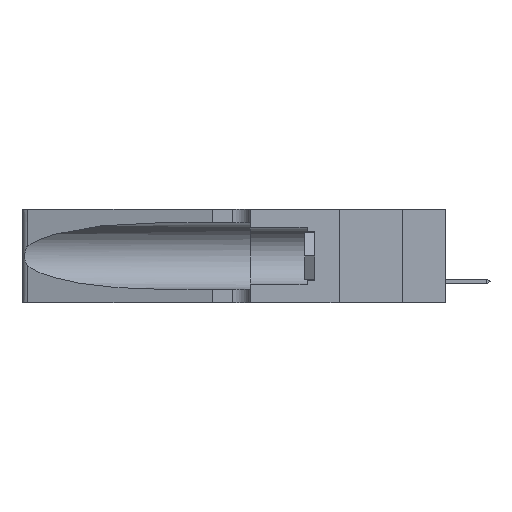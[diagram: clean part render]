
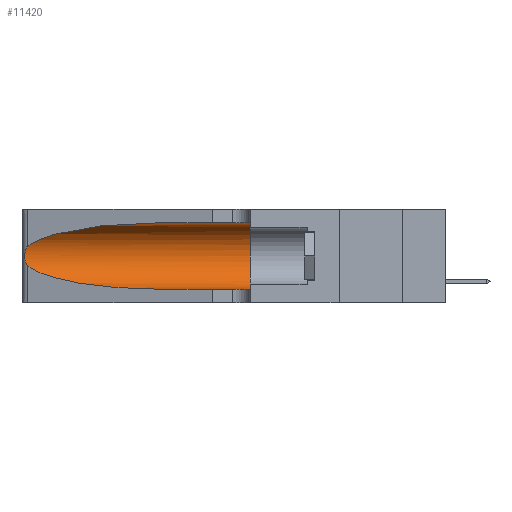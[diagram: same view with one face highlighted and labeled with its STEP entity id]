
A CAD part, left-side view. The second image highlights one B-rep face of the part: STEP entity #11420.
In plain terms, the highlighted cylindrical face has radius 3.308 mm (diameter 6.617 mm), a partial arc.
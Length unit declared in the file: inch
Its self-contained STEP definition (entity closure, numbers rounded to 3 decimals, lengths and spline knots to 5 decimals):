
#51 = EDGE_CURVE ( 'NONE', #38348, #25150, #23534, .T. ) ;
#70 = AXIS2_PLACEMENT_3D ( 'NONE', #29492, #16623, #16919 ) ;
#485 =( BOUNDED_CURVE ( )  B_SPLINE_CURVE ( 3, ( #26057, #1219, #16881, #4273 ),
 .UNSPECIFIED., .F., .F. ) 
 B_SPLINE_CURVE_WITH_KNOTS ( ( 4, 4 ),
 ( 1.5708, 2.84003 ),
 .UNSPECIFIED. ) 
 CURVE ( )  GEOMETRIC_REPRESENTATION_ITEM ( )  RATIONAL_B_SPLINE_CURVE ( ( 1., 0.87, 0.87, 1. ) ) 
 REPRESENTATION_ITEM ( '' )  );
#1219 = CARTESIAN_POINT ( 'NONE',  ( 0.18966, 0.96281, 0.31525 ) ) ;
#1238 = DIRECTION ( 'NONE',  ( 0., 0., 1. ) ) ;
#1259 = CARTESIAN_POINT ( 'NONE',  ( 0.25487, 1.22718, 0.14631 ) ) ;
#2976 = DIRECTION ( 'NONE',  ( 0., -1., 0. ) ) ;
#3094 = CARTESIAN_POINT ( 'NONE',  ( 0.2373, 1.15595, 0.08982 ) ) ;
#3596 = CARTESIAN_POINT ( 'NONE',  ( 0.1305, 0.72297, 0.05475 ) ) ;
#3886 = EDGE_CURVE ( 'NONE', #4563, #26583, #12481, .T. ) ;
#4153 = VECTOR ( 'NONE', #2976, 39.37008 ) ;
#4273 = CARTESIAN_POINT ( 'NONE',  ( 0.25487, 1.22718, 0.22369 ) ) ;
#4319 = CIRCLE ( 'NONE', #8875, 0.13025 ) ;
#4563 = VERTEX_POINT ( 'NONE', #3596 ) ;
#4903 = CARTESIAN_POINT ( 'NONE',  ( 0.25487, 1.22718, 0.22369 ) ) ;
#5535 = ORIENTED_EDGE ( 'NONE', *, *, #51, .F. ) ;
#6476 = ORIENTED_EDGE ( 'NONE', *, *, #31259, .T. ) ;
#6793 = FACE_OUTER_BOUND ( 'NONE', #39763, .T. ) ;
#7036 =( BOUNDED_CURVE ( )  B_SPLINE_CURVE ( 3, ( #18061, #3094, #12123, #31161 ),
 .UNSPECIFIED., .F., .T. ) 
 B_SPLINE_CURVE_WITH_KNOTS ( ( 4, 4 ),
 ( 3.44316, 4.71239 ),
 .UNSPECIFIED. ) 
 CURVE ( )  GEOMETRIC_REPRESENTATION_ITEM ( )  RATIONAL_B_SPLINE_CURVE ( ( 1., 0.87, 0.87, 1. ) ) 
 REPRESENTATION_ITEM ( '' )  );
#7066 = EDGE_CURVE ( 'NONE', #38348, #38862, #485, .T. ) ;
#8541 = CARTESIAN_POINT ( 'NONE',  ( 0.25787, 1.23484, 0.2124 ) ) ;
#8875 = AXIS2_PLACEMENT_3D ( 'NONE', #19814, #23179, #1238 ) ;
#10843 = CARTESIAN_POINT ( 'NONE',  ( 0.1305, 0.35, 0.05475 ) ) ;
#11185 = ORIENTED_EDGE ( 'NONE', *, *, #7066, .T. ) ;
#11324 = CARTESIAN_POINT ( 'NONE',  ( 0.25854, 1.2359, 0.20912 ) ) ;
#11420 = ADVANCED_FACE ( 'NONE', ( #6793 ), #32430, .F. ) ;
#11599 = CARTESIAN_POINT ( 'NONE',  ( 0.25789, 1.23486, 0.15765 ) ) ;
#11726 = CARTESIAN_POINT ( 'NONE',  ( 0.26075, 1.23896, 0.178 ) ) ;
#12123 = CARTESIAN_POINT ( 'NONE',  ( 0.18966, 0.96281, 0.05475 ) ) ;
#12189 = CARTESIAN_POINT ( 'NONE',  ( 0.1305, 0.35, 0.31525 ) ) ;
#12481 = LINE ( 'NONE', #31179, #4153 ) ;
#14331 = CARTESIAN_POINT ( 'NONE',  ( 0.25555, 1.22994, 0.2215 ) ) ;
#14461 = CARTESIAN_POINT ( 'NONE',  ( 0.25487, 1.22718, 0.14631 ) ) ;
#15087 = VECTOR ( 'NONE', #19392, 39.37008 ) ;
#16623 = DIRECTION ( 'NONE',  ( 0., -1., 0. ) ) ;
#16881 = CARTESIAN_POINT ( 'NONE',  ( 0.2373, 1.15595, 0.28018 ) ) ;
#16919 = DIRECTION ( 'NONE',  ( 0., 0., -1. ) ) ;
#17799 = CARTESIAN_POINT ( 'NONE',  ( 0.1305, 0.72297, 0.31525 ) ) ;
#18061 = CARTESIAN_POINT ( 'NONE',  ( 0.25487, 1.22718, 0.14631 ) ) ;
#18264 = EDGE_CURVE ( 'NONE', #38862, #28192, #24837, .T. ) ;
#18479 = ORIENTED_EDGE ( 'NONE', *, *, #31520, .F. ) ;
#19392 = DIRECTION ( 'NONE',  ( 0., -1., 0. ) ) ;
#19814 = CARTESIAN_POINT ( 'NONE',  ( 0.1305, 0.35, 0.185 ) ) ;
#21139 = CARTESIAN_POINT ( 'NONE',  ( 0.26075, 1.23896, 0.19203 ) ) ;
#23179 = DIRECTION ( 'NONE',  ( 0., 1., 0. ) ) ;
#23534 = LINE ( 'NONE', #31944, #15087 ) ;
#24211 = CARTESIAN_POINT ( 'NONE',  ( 0.25639, 1.23186, 0.15144 ) ) ;
#24837 = B_SPLINE_CURVE_WITH_KNOTS ( 'NONE', 3,
 ( #4903, #14331, #39460, #8541, #11324, #36428, #21139, #11726, #33386, #36843, #11599, #24211, #33784, #14461 ),
 .UNSPECIFIED., .F., .F.,
 ( 4, 2, 2, 2, 2, 2, 4 ),
 ( 0., 0.00027, 0.00053, 0.00107, 0.0016, 0.00187, 0.00214 ),
 .UNSPECIFIED. ) ;
#25150 = VERTEX_POINT ( 'NONE', #12189 ) ;
#26057 = CARTESIAN_POINT ( 'NONE',  ( 0.1305, 0.72297, 0.31525 ) ) ;
#26583 = VERTEX_POINT ( 'NONE', #10843 ) ;
#28192 = VERTEX_POINT ( 'NONE', #1259 ) ;
#29492 = CARTESIAN_POINT ( 'NONE',  ( 0.1305, 1.61858, 0.185 ) ) ;
#30539 = ORIENTED_EDGE ( 'NONE', *, *, #18264, .T. ) ;
#31161 = CARTESIAN_POINT ( 'NONE',  ( 0.1305, 0.72297, 0.05475 ) ) ;
#31179 = CARTESIAN_POINT ( 'NONE',  ( 0.1305, 1.61858, 0.05475 ) ) ;
#31259 = EDGE_CURVE ( 'NONE', #28192, #4563, #7036, .T. ) ;
#31520 = EDGE_CURVE ( 'NONE', #25150, #26583, #4319, .T. ) ;
#31944 = CARTESIAN_POINT ( 'NONE',  ( 0.1305, 1.61858, 0.31525 ) ) ;
#32430 = CYLINDRICAL_SURFACE ( 'NONE', #70, 0.13025 ) ;
#33386 = CARTESIAN_POINT ( 'NONE',  ( 0.26017, 1.23833, 0.17102 ) ) ;
#33784 = CARTESIAN_POINT ( 'NONE',  ( 0.25555, 1.22993, 0.14849 ) ) ;
#36141 = CARTESIAN_POINT ( 'NONE',  ( 0.25487, 1.22718, 0.22369 ) ) ;
#36428 = CARTESIAN_POINT ( 'NONE',  ( 0.26018, 1.23835, 0.19895 ) ) ;
#36843 = CARTESIAN_POINT ( 'NONE',  ( 0.25856, 1.23593, 0.16098 ) ) ;
#38348 = VERTEX_POINT ( 'NONE', #17799 ) ;
#38862 = VERTEX_POINT ( 'NONE', #36141 ) ;
#39460 = CARTESIAN_POINT ( 'NONE',  ( 0.25639, 1.23184, 0.21858 ) ) ;
#39763 = EDGE_LOOP ( 'NONE', ( #11185, #30539, #6476, #40827, #18479, #5535 ) ) ;
#40827 = ORIENTED_EDGE ( 'NONE', *, *, #3886, .T. ) ;
